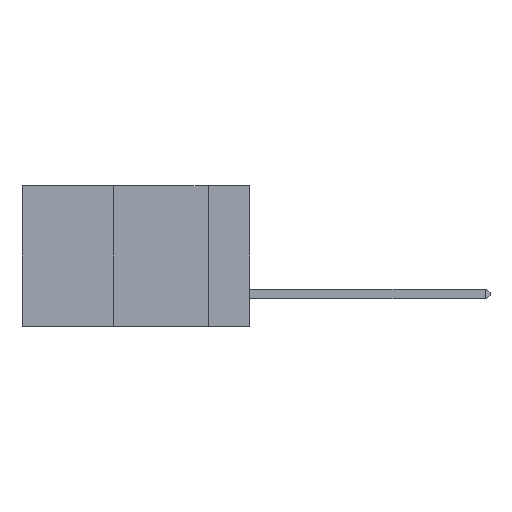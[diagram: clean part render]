
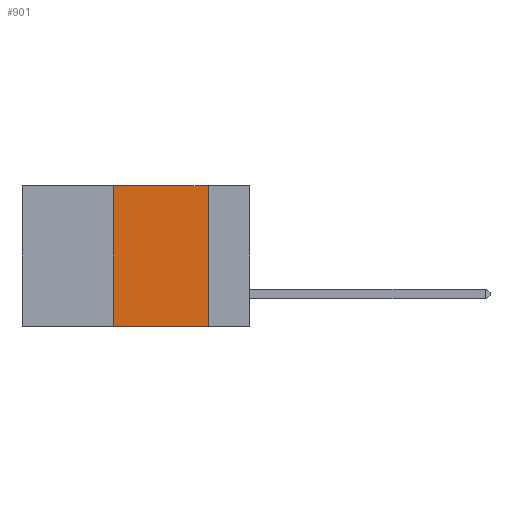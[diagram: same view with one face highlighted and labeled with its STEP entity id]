
A CAD part, left-side view. The second image highlights one B-rep face of the part: STEP entity #901.
In plain terms, the highlighted planar face has unit normal (-1, 0, 0).
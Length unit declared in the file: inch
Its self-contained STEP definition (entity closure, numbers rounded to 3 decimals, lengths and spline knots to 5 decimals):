
#17 = VERTEX_POINT ( 'NONE', #4815 ) ;
#137 = EDGE_CURVE ( 'NONE', #17, #9695, #8991, .T. ) ;
#273 = VECTOR ( 'NONE', #10229, 39.37008 ) ;
#568 = LINE ( 'NONE', #9502, #273 ) ;
#691 = PLANE ( 'NONE',  #2374 ) ;
#901 = ADVANCED_FACE ( 'NONE', ( #1599 ), #691, .F. ) ;
#1489 = EDGE_LOOP ( 'NONE', ( #2729, #3392, #4113, #1881 ) ) ;
#1599 = FACE_OUTER_BOUND ( 'NONE', #1489, .T. ) ;
#1881 = ORIENTED_EDGE ( 'NONE', *, *, #7270, .T. ) ;
#1923 = CARTESIAN_POINT ( 'NONE',  ( 0., 0.6, 0. ) ) ;
#2373 = DIRECTION ( 'NONE',  ( 1., 0., 0. ) ) ;
#2374 = AXIS2_PLACEMENT_3D ( 'NONE', #1923, #2373, #3111 ) ;
#2729 = ORIENTED_EDGE ( 'NONE', *, *, #137, .F. ) ;
#3009 = VERTEX_POINT ( 'NONE', #8246 ) ;
#3111 = DIRECTION ( 'NONE',  ( 0., 0., -1. ) ) ;
#3392 = ORIENTED_EDGE ( 'NONE', *, *, #10012, .F. ) ;
#4113 = ORIENTED_EDGE ( 'NONE', *, *, #10643, .F. ) ;
#4163 = DIRECTION ( 'NONE',  ( 0., 0., -1. ) ) ;
#4815 = CARTESIAN_POINT ( 'NONE',  ( 0., 0.11, 0. ) ) ;
#5206 = LINE ( 'NONE', #9582, #9463 ) ;
#5397 = LINE ( 'NONE', #7571, #7067 ) ;
#5616 = DIRECTION ( 'NONE',  ( 0., -1., 0. ) ) ;
#6536 = DIRECTION ( 'NONE',  ( 0., -1., 0. ) ) ;
#6854 = VECTOR ( 'NONE', #4163, 39.37008 ) ;
#7067 = VECTOR ( 'NONE', #6536, 39.37008 ) ;
#7270 = EDGE_CURVE ( 'NONE', #3009, #9695, #5397, .T. ) ;
#7571 = CARTESIAN_POINT ( 'NONE',  ( 0., 0.6, -0.37 ) ) ;
#7646 = CARTESIAN_POINT ( 'NONE',  ( 0., 0.11, -0.37 ) ) ;
#8246 = CARTESIAN_POINT ( 'NONE',  ( 0., 0.36, -0.37 ) ) ;
#8269 = CARTESIAN_POINT ( 'NONE',  ( 0., 0.11, 0. ) ) ;
#8550 = VERTEX_POINT ( 'NONE', #10018 ) ;
#8991 = LINE ( 'NONE', #8269, #6854 ) ;
#9463 = VECTOR ( 'NONE', #5616, 39.37008 ) ;
#9502 = CARTESIAN_POINT ( 'NONE',  ( 0., 0.36, 0. ) ) ;
#9582 = CARTESIAN_POINT ( 'NONE',  ( 0., 0.6, 0. ) ) ;
#9695 = VERTEX_POINT ( 'NONE', #7646 ) ;
#10012 = EDGE_CURVE ( 'NONE', #8550, #17, #5206, .T. ) ;
#10018 = CARTESIAN_POINT ( 'NONE',  ( 0., 0.36, 0. ) ) ;
#10229 = DIRECTION ( 'NONE',  ( 0., 0., 1. ) ) ;
#10643 = EDGE_CURVE ( 'NONE', #3009, #8550, #568, .T. ) ;
